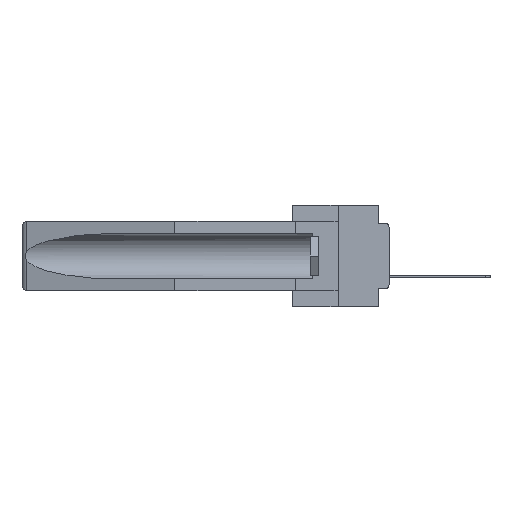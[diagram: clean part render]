
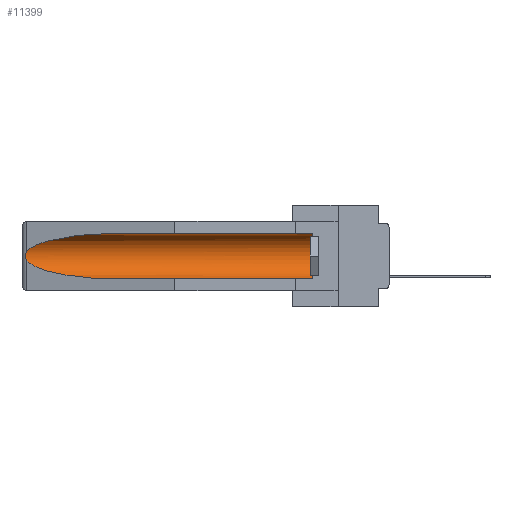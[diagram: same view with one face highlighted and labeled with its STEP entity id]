
A CAD part, left-side view. The second image highlights one B-rep face of the part: STEP entity #11399.
In plain terms, the highlighted cylindrical face has radius 2.857 mm (diameter 5.715 mm), a partial arc.
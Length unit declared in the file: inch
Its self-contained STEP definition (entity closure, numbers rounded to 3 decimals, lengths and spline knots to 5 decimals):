
#345 = DIRECTION ( 'NONE',  ( 0., 1., 0. ) ) ;
#2252 = CARTESIAN_POINT ( 'NONE',  ( 0.155, 0.126, -0.059 ) ) ;
#3759 = VERTEX_POINT ( 'NONE', #2252 ) ;
#3912 = ORIENTED_EDGE ( 'NONE', *, *, #18004, .T. ) ;
#4265 = CYLINDRICAL_SURFACE ( 'NONE', #25618, 0.1125 ) ;
#4367 = CARTESIAN_POINT ( 'NONE',  ( 0.26597, 1.52961, -0.15275 ) ) ;
#5023 = LINE ( 'NONE', #12314, #10777 ) ;
#5514 = CARTESIAN_POINT ( 'NONE',  ( 0.155, 1.07973, -0.284 ) ) ;
#5831 = CARTESIAN_POINT ( 'NONE',  ( 0.26537, 1.52718, -0.14972 ) ) ;
#6001 = ORIENTED_EDGE ( 'NONE', *, *, #26162, .T. ) ;
#6342 = VECTOR ( 'NONE', #345, 39.37008 ) ;
#6378 = CARTESIAN_POINT ( 'NONE',  ( 0.2673, 1.5327, -0.16383 ) ) ;
#6478 = CARTESIAN_POINT ( 'NONE',  ( 0.2675, 1.53308, -0.17534 ) ) ;
#7322 = CARTESIAN_POINT ( 'NONE',  ( 0.155, -0.30754, -0.1715 ) ) ;
#7714 = EDGE_CURVE ( 'NONE', #29391, #3759, #19458, .T. ) ;
#8264 = AXIS2_PLACEMENT_3D ( 'NONE', #15492, #15584, #27365 ) ;
#8463 = CARTESIAN_POINT ( 'NONE',  ( 0.2673, 1.53269, -0.17917 ) ) ;
#8754 = CARTESIAN_POINT ( 'NONE',  ( 0.2675, 1.53308, -0.16763 ) ) ;
#9660 = CARTESIAN_POINT ( 'NONE',  ( 0.26537, 1.52718, -0.14972 ) ) ;
#10400 = CARTESIAN_POINT ( 'NONE',  ( 0.155, 1.07973, -0.059 ) ) ;
#10769 = CARTESIAN_POINT ( 'NONE',  ( 0.26597, 1.5296, -0.19026 ) ) ;
#10777 = VECTOR ( 'NONE', #26494, 39.37008 ) ;
#10825 = CARTESIAN_POINT ( 'NONE',  ( 0.155, 1.07973, -0.284 ) ) ;
#11399 = ADVANCED_FACE ( 'NONE', ( #28265 ), #4265, .F. ) ;
#11866 = CARTESIAN_POINT ( 'NONE',  ( 0.21114, 1.30732, -0.059 ) ) ;
#11991 = DIRECTION ( 'NONE',  ( 0., 0., 1. ) ) ;
#12109 = VERTEX_POINT ( 'NONE', #5514 ) ;
#12314 = CARTESIAN_POINT ( 'NONE',  ( 0.155, -0.30754, -0.284 ) ) ;
#12944 = ORIENTED_EDGE ( 'NONE', *, *, #26492, .T. ) ;
#15201 = CARTESIAN_POINT ( 'NONE',  ( 0.26537, 1.52718, -0.19328 ) ) ;
#15492 = CARTESIAN_POINT ( 'NONE',  ( 0.155, 0.126, -0.1715 ) ) ;
#15584 = DIRECTION ( 'NONE',  ( 0., -1., 0. ) ) ;
#15647 = CARTESIAN_POINT ( 'NONE',  ( 0.26655, 1.53094, -0.18657 ) ) ;
#16352 = ORIENTED_EDGE ( 'NONE', *, *, #7714, .T. ) ;
#16641 = CARTESIAN_POINT ( 'NONE',  ( 0.25451, 1.48313, -0.09465 ) ) ;
#16749 = VERTEX_POINT ( 'NONE', #5831 ) ;
#18004 = EDGE_CURVE ( 'NONE', #25548, #12109, #25296, .T. ) ;
#18037 = CARTESIAN_POINT ( 'NONE',  ( 0.26537, 1.52718, -0.14972 ) ) ;
#18072 =( BOUNDED_CURVE ( )  B_SPLINE_CURVE ( 3, ( #23329, #11866, #16641, #9660 ),
 .UNSPECIFIED., .F., .F. ) 
 B_SPLINE_CURVE_WITH_KNOTS ( ( 4, 4 ),
 ( 4.71239, 6.08839 ),
 .UNSPECIFIED. ) 
 CURVE ( )  GEOMETRIC_REPRESENTATION_ITEM ( )  RATIONAL_B_SPLINE_CURVE ( ( 1., 0.848, 0.848, 1. ) ) 
 REPRESENTATION_ITEM ( '' )  );
#19458 = CIRCLE ( 'NONE', #8264, 0.1125 ) ;
#21089 = CARTESIAN_POINT ( 'NONE',  ( 0.155, 0.126, -0.284 ) ) ;
#21490 = CARTESIAN_POINT ( 'NONE',  ( 0.26537, 1.52718, -0.19328 ) ) ;
#21765 = EDGE_CURVE ( 'NONE', #16749, #25548, #27860, .T. ) ;
#22284 = CARTESIAN_POINT ( 'NONE',  ( 0.21114, 1.30732, -0.284 ) ) ;
#22285 = ORIENTED_EDGE ( 'NONE', *, *, #29498, .F. ) ;
#22438 = CARTESIAN_POINT ( 'NONE',  ( 0.26537, 1.52718, -0.19328 ) ) ;
#22766 = VERTEX_POINT ( 'NONE', #10400 ) ;
#22859 = LINE ( 'NONE', #25863, #6342 ) ;
#23329 = CARTESIAN_POINT ( 'NONE',  ( 0.155, 1.07973, -0.059 ) ) ;
#23611 = EDGE_LOOP ( 'NONE', ( #12944, #27813, #3912, #22285, #16352, #6001 ) ) ;
#25296 =( BOUNDED_CURVE ( )  B_SPLINE_CURVE ( 3, ( #15201, #26801, #22284, #10825 ),
 .UNSPECIFIED., .F., .F. ) 
 B_SPLINE_CURVE_WITH_KNOTS ( ( 4, 4 ),
 ( 0.1948, 1.5708 ),
 .UNSPECIFIED. ) 
 CURVE ( )  GEOMETRIC_REPRESENTATION_ITEM ( )  RATIONAL_B_SPLINE_CURVE ( ( 1., 0.848, 0.848, 1. ) ) 
 REPRESENTATION_ITEM ( '' )  );
#25548 = VERTEX_POINT ( 'NONE', #21490 ) ;
#25618 = AXIS2_PLACEMENT_3D ( 'NONE', #7322, #28105, #11991 ) ;
#25863 = CARTESIAN_POINT ( 'NONE',  ( 0.155, -0.30754, -0.059 ) ) ;
#26162 = EDGE_CURVE ( 'NONE', #3759, #22766, #22859, .T. ) ;
#26492 = EDGE_CURVE ( 'NONE', #22766, #16749, #18072, .T. ) ;
#26494 = DIRECTION ( 'NONE',  ( 0., 1., 0. ) ) ;
#26801 = CARTESIAN_POINT ( 'NONE',  ( 0.25451, 1.48313, -0.24835 ) ) ;
#26855 = CARTESIAN_POINT ( 'NONE',  ( 0.26654, 1.53092, -0.15636 ) ) ;
#27365 = DIRECTION ( 'NONE',  ( 0., 0., 1. ) ) ;
#27813 = ORIENTED_EDGE ( 'NONE', *, *, #21765, .T. ) ;
#27860 = B_SPLINE_CURVE_WITH_KNOTS ( 'NONE', 3,
 ( #18037, #4367, #26855, #6378, #8754, #6478, #8463, #15647, #10769, #22438 ),
 .UNSPECIFIED., .F., .F.,
 ( 4, 2, 2, 2, 4 ),
 ( 0., 0.00029, 0.00058, 0.00087, 0.00117 ),
 .UNSPECIFIED. ) ;
#28105 = DIRECTION ( 'NONE',  ( 0., 1., 0. ) ) ;
#28265 = FACE_OUTER_BOUND ( 'NONE', #23611, .T. ) ;
#29391 = VERTEX_POINT ( 'NONE', #21089 ) ;
#29498 = EDGE_CURVE ( 'NONE', #29391, #12109, #5023, .T. ) ;
